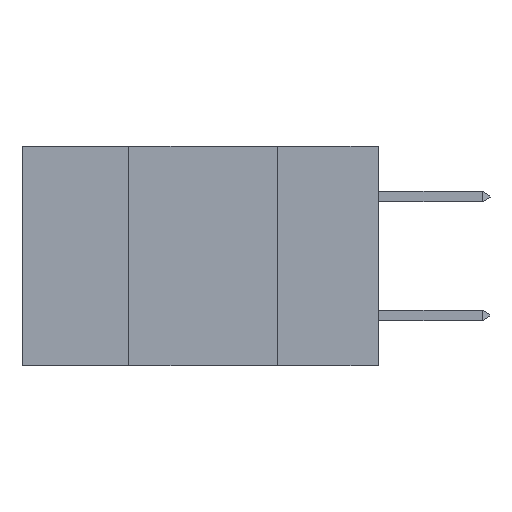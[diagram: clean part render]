
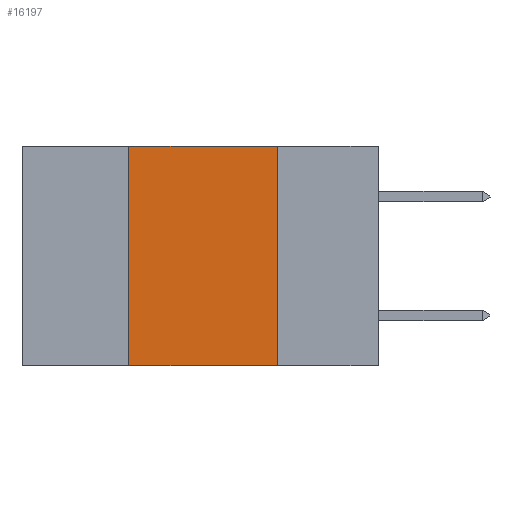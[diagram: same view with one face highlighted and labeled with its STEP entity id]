
A CAD part, left-side view. The second image highlights one B-rep face of the part: STEP entity #16197.
In plain terms, the highlighted planar face has unit normal (-1, 0, 0).
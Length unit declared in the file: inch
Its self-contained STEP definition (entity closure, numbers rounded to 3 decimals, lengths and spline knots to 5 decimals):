
#2435 = VECTOR ( 'NONE', #13935, 39.37008 ) ;
#2482 = CARTESIAN_POINT ( 'NONE',  ( 0., 0.6, 0. ) ) ;
#2795 = FACE_OUTER_BOUND ( 'NONE', #29089, .T. ) ;
#3470 = CARTESIAN_POINT ( 'NONE',  ( 0., 0.6, -0.37 ) ) ;
#3505 = VECTOR ( 'NONE', #17292, 39.37008 ) ;
#3591 = VERTEX_POINT ( 'NONE', #30659 ) ;
#3863 = LINE ( 'NONE', #24997, #28960 ) ;
#5273 = ORIENTED_EDGE ( 'NONE', *, *, #26393, .F. ) ;
#6804 = ORIENTED_EDGE ( 'NONE', *, *, #9680, .F. ) ;
#7394 = DIRECTION ( 'NONE',  ( 1., 0., 0. ) ) ;
#9680 = EDGE_CURVE ( 'NONE', #16265, #23301, #15530, .T. ) ;
#12962 = ORIENTED_EDGE ( 'NONE', *, *, #17735, .F. ) ;
#13935 = DIRECTION ( 'NONE',  ( 0., 0., -1. ) ) ;
#13981 = VERTEX_POINT ( 'NONE', #18303 ) ;
#14751 = PLANE ( 'NONE',  #21163 ) ;
#14836 = CARTESIAN_POINT ( 'NONE',  ( 0., 0.6, 0. ) ) ;
#15072 = CARTESIAN_POINT ( 'NONE',  ( 0., 0.17, 0. ) ) ;
#15486 = VECTOR ( 'NONE', #20558, 39.37008 ) ;
#15530 = LINE ( 'NONE', #28310, #2435 ) ;
#16197 = ADVANCED_FACE ( 'NONE', ( #2795 ), #14751, .F. ) ;
#16265 = VERTEX_POINT ( 'NONE', #15072 ) ;
#16454 = EDGE_CURVE ( 'NONE', #13981, #23301, #28317, .T. ) ;
#17292 = DIRECTION ( 'NONE',  ( 0., -1., 0. ) ) ;
#17735 = EDGE_CURVE ( 'NONE', #13981, #3591, #3863, .T. ) ;
#18303 = CARTESIAN_POINT ( 'NONE',  ( 0., 0.42, -0.37 ) ) ;
#19790 = ORIENTED_EDGE ( 'NONE', *, *, #16454, .T. ) ;
#20558 = DIRECTION ( 'NONE',  ( 0., -1., 0. ) ) ;
#21163 = AXIS2_PLACEMENT_3D ( 'NONE', #2482, #7394, #24484 ) ;
#22642 = DIRECTION ( 'NONE',  ( 0., 0., 1. ) ) ;
#22850 = CARTESIAN_POINT ( 'NONE',  ( 0., 0.17, -0.37 ) ) ;
#22959 = LINE ( 'NONE', #14836, #3505 ) ;
#23301 = VERTEX_POINT ( 'NONE', #22850 ) ;
#24484 = DIRECTION ( 'NONE',  ( 0., 0., -1. ) ) ;
#24997 = CARTESIAN_POINT ( 'NONE',  ( 0., 0.42, 0. ) ) ;
#26393 = EDGE_CURVE ( 'NONE', #3591, #16265, #22959, .T. ) ;
#28310 = CARTESIAN_POINT ( 'NONE',  ( 0., 0.17, 0. ) ) ;
#28317 = LINE ( 'NONE', #3470, #15486 ) ;
#28960 = VECTOR ( 'NONE', #22642, 39.37008 ) ;
#29089 = EDGE_LOOP ( 'NONE', ( #6804, #5273, #12962, #19790 ) ) ;
#30659 = CARTESIAN_POINT ( 'NONE',  ( 0., 0.42, 0. ) ) ;
